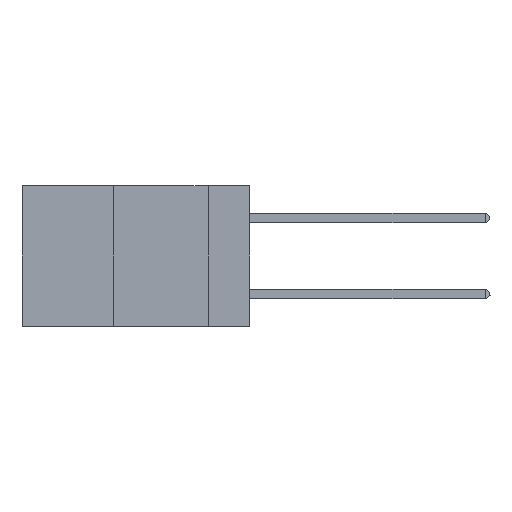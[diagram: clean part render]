
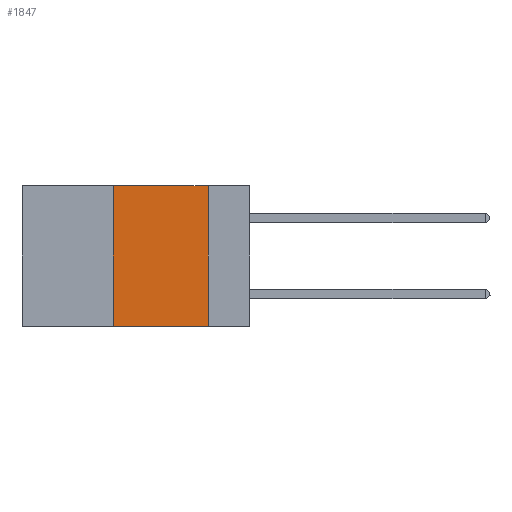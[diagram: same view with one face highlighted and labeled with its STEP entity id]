
A CAD part, left-side view. The second image highlights one B-rep face of the part: STEP entity #1847.
In plain terms, the highlighted planar face has unit normal (-1, 0, 0).
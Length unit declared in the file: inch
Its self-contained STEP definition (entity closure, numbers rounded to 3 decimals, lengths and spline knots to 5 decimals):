
#34 = CARTESIAN_POINT ( 'NONE',  ( 0., 0.36, 0. ) ) ;
#457 = DIRECTION ( 'NONE',  ( 0., -1., 0. ) ) ;
#1201 = VECTOR ( 'NONE', #6746, 39.37008 ) ;
#1215 = CARTESIAN_POINT ( 'NONE',  ( 0., 0.11, -0.37 ) ) ;
#1568 = ORIENTED_EDGE ( 'NONE', *, *, #10114, .T. ) ;
#1580 = CARTESIAN_POINT ( 'NONE',  ( 0., 0.6, 0. ) ) ;
#1590 = VERTEX_POINT ( 'NONE', #1215 ) ;
#1847 = ADVANCED_FACE ( 'NONE', ( #5303 ), #6406, .F. ) ;
#2594 = ORIENTED_EDGE ( 'NONE', *, *, #10991, .F. ) ;
#2614 = DIRECTION ( 'NONE',  ( 0., 0., -1. ) ) ;
#3408 = CARTESIAN_POINT ( 'NONE',  ( 0., 0.11, 0. ) ) ;
#3532 = ORIENTED_EDGE ( 'NONE', *, *, #6471, .F. ) ;
#4132 = EDGE_LOOP ( 'NONE', ( #11868, #2594, #3532, #1568 ) ) ;
#4155 = VECTOR ( 'NONE', #10302, 39.37008 ) ;
#5303 = FACE_OUTER_BOUND ( 'NONE', #4132, .T. ) ;
#6240 = LINE ( 'NONE', #10152, #4155 ) ;
#6359 = DIRECTION ( 'NONE',  ( 1., 0., 0. ) ) ;
#6406 = PLANE ( 'NONE',  #7744 ) ;
#6471 = EDGE_CURVE ( 'NONE', #8751, #6887, #10367, .T. ) ;
#6746 = DIRECTION ( 'NONE',  ( 0., -1., 0. ) ) ;
#6887 = VERTEX_POINT ( 'NONE', #34 ) ;
#6939 = CARTESIAN_POINT ( 'NONE',  ( 0., 0.36, 0. ) ) ;
#7103 = CARTESIAN_POINT ( 'NONE',  ( 0., 0.6, 0. ) ) ;
#7136 = LINE ( 'NONE', #9515, #1201 ) ;
#7744 = AXIS2_PLACEMENT_3D ( 'NONE', #1580, #6359, #2614 ) ;
#7873 = DIRECTION ( 'NONE',  ( 0., 0., 1. ) ) ;
#8150 = VECTOR ( 'NONE', #7873, 39.37008 ) ;
#8751 = VERTEX_POINT ( 'NONE', #9010 ) ;
#9010 = CARTESIAN_POINT ( 'NONE',  ( 0., 0.36, -0.37 ) ) ;
#9450 = VECTOR ( 'NONE', #457, 39.37008 ) ;
#9515 = CARTESIAN_POINT ( 'NONE',  ( 0., 0.6, -0.37 ) ) ;
#9898 = LINE ( 'NONE', #7103, #9450 ) ;
#9938 = EDGE_CURVE ( 'NONE', #11933, #1590, #6240, .T. ) ;
#10114 = EDGE_CURVE ( 'NONE', #8751, #1590, #7136, .T. ) ;
#10152 = CARTESIAN_POINT ( 'NONE',  ( 0., 0.11, 0. ) ) ;
#10302 = DIRECTION ( 'NONE',  ( 0., 0., -1. ) ) ;
#10367 = LINE ( 'NONE', #6939, #8150 ) ;
#10991 = EDGE_CURVE ( 'NONE', #6887, #11933, #9898, .T. ) ;
#11868 = ORIENTED_EDGE ( 'NONE', *, *, #9938, .F. ) ;
#11933 = VERTEX_POINT ( 'NONE', #3408 ) ;
